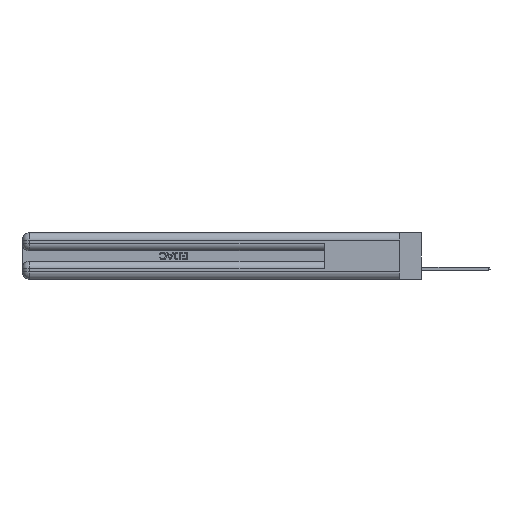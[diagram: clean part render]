
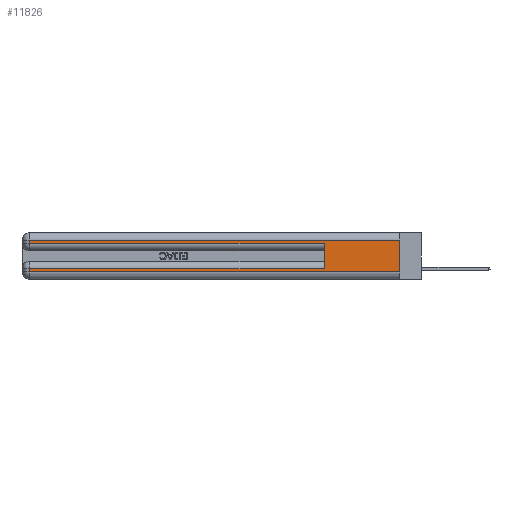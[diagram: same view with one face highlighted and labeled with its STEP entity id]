
A CAD part, left-side view. The second image highlights one B-rep face of the part: STEP entity #11826.
In plain terms, the highlighted planar face has unit normal (-1, 0, 0).
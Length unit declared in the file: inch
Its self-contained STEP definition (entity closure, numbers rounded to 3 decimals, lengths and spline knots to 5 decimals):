
#7 = VECTOR ( 'NONE', #46256, 39.37008 ) ;
#657 = VERTEX_POINT ( 'NONE', #34122 ) ;
#1101 = VECTOR ( 'NONE', #44499, 39.37008 ) ;
#2523 = EDGE_LOOP ( 'NONE', ( #15719, #14985, #14966, #12676, #46068, #41297, #9200, #43063 ) ) ;
#3746 = CARTESIAN_POINT ( 'NONE',  ( 0., 2.94, 0.37 ) ) ;
#4333 = CARTESIAN_POINT ( 'NONE',  ( 0., 0.6, 0.145 ) ) ;
#4435 = VECTOR ( 'NONE', #31436, 39.37008 ) ;
#6180 = VECTOR ( 'NONE', #40109, 39.37008 ) ;
#6723 = VERTEX_POINT ( 'NONE', #40506 ) ;
#6785 = DIRECTION ( 'NONE',  ( 1., 0., 0. ) ) ;
#7247 = CARTESIAN_POINT ( 'NONE',  ( 0., 0., 0.285 ) ) ;
#8791 = CARTESIAN_POINT ( 'NONE',  ( 0., 0.6, 0.285 ) ) ;
#9200 = ORIENTED_EDGE ( 'NONE', *, *, #17586, .T. ) ;
#10290 = CARTESIAN_POINT ( 'NONE',  ( 0., 2.94, 0.37 ) ) ;
#10808 = EDGE_CURVE ( 'NONE', #46349, #21375, #18232, .T. ) ;
#11057 = DIRECTION ( 'NONE',  ( 0., -1., 0. ) ) ;
#11526 = AXIS2_PLACEMENT_3D ( 'NONE', #44281, #6785, #19228 ) ;
#11826 = ADVANCED_FACE ( 'NONE', ( #45069 ), #40083, .F. ) ;
#12674 = CARTESIAN_POINT ( 'NONE',  ( 0., 0., 0.37 ) ) ;
#12676 = ORIENTED_EDGE ( 'NONE', *, *, #21473, .T. ) ;
#13529 = CARTESIAN_POINT ( 'NONE',  ( 0., 0., 0.31 ) ) ;
#14966 = ORIENTED_EDGE ( 'NONE', *, *, #46857, .T. ) ;
#14985 = ORIENTED_EDGE ( 'NONE', *, *, #49122, .T. ) ;
#15719 = ORIENTED_EDGE ( 'NONE', *, *, #10808, .F. ) ;
#16898 = LINE ( 'NONE', #32033, #4435 ) ;
#17586 = EDGE_CURVE ( 'NONE', #51857, #6723, #37594, .T. ) ;
#18232 = LINE ( 'NONE', #12674, #7 ) ;
#18867 = CARTESIAN_POINT ( 'NONE',  ( 0., 2.94, 0.31 ) ) ;
#19228 = DIRECTION ( 'NONE',  ( 0., 0., -1. ) ) ;
#21375 = VERTEX_POINT ( 'NONE', #40155 ) ;
#21473 = EDGE_CURVE ( 'NONE', #45575, #36614, #45914, .T. ) ;
#22296 = EDGE_CURVE ( 'NONE', #6723, #21375, #43138, .T. ) ;
#23285 = LINE ( 'NONE', #23460, #6180 ) ;
#23460 = CARTESIAN_POINT ( 'NONE',  ( 0., 0., 0.31 ) ) ;
#25037 = LINE ( 'NONE', #4333, #49140 ) ;
#25168 = DIRECTION ( 'NONE',  ( 0., 0., -1. ) ) ;
#30613 = VECTOR ( 'NONE', #39414, 39.37008 ) ;
#31436 = DIRECTION ( 'NONE',  ( 0., 1., 0. ) ) ;
#32033 = CARTESIAN_POINT ( 'NONE',  ( 0., 0., 0.085 ) ) ;
#34122 = CARTESIAN_POINT ( 'NONE',  ( 0., 0.6, 0.085 ) ) ;
#35729 = CARTESIAN_POINT ( 'NONE',  ( 0., 0., 0.06 ) ) ;
#36614 = VERTEX_POINT ( 'NONE', #8791 ) ;
#37306 = CARTESIAN_POINT ( 'NONE',  ( 0., 2.94, 0.285 ) ) ;
#37594 = LINE ( 'NONE', #3746, #42109 ) ;
#39414 = DIRECTION ( 'NONE',  ( 0., 0., -1. ) ) ;
#39832 = EDGE_CURVE ( 'NONE', #657, #36614, #25037, .T. ) ;
#40083 = PLANE ( 'NONE',  #11526 ) ;
#40109 = DIRECTION ( 'NONE',  ( 0., 1., 0. ) ) ;
#40155 = CARTESIAN_POINT ( 'NONE',  ( 0., 0., 0.06 ) ) ;
#40506 = CARTESIAN_POINT ( 'NONE',  ( 0., 2.94, 0.06 ) ) ;
#41127 = CARTESIAN_POINT ( 'NONE',  ( 0., 2.94, 0.085 ) ) ;
#41297 = ORIENTED_EDGE ( 'NONE', *, *, #41878, .T. ) ;
#41878 = EDGE_CURVE ( 'NONE', #657, #51857, #16898, .T. ) ;
#42109 = VECTOR ( 'NONE', #25168, 39.37008 ) ;
#43063 = ORIENTED_EDGE ( 'NONE', *, *, #22296, .T. ) ;
#43138 = LINE ( 'NONE', #35729, #1101 ) ;
#44281 = CARTESIAN_POINT ( 'NONE',  ( 0., 0., 0.37 ) ) ;
#44499 = DIRECTION ( 'NONE',  ( 0., -1., 0. ) ) ;
#45069 = FACE_OUTER_BOUND ( 'NONE', #2523, .T. ) ;
#45324 = VECTOR ( 'NONE', #11057, 39.37008 ) ;
#45575 = VERTEX_POINT ( 'NONE', #37306 ) ;
#45914 = LINE ( 'NONE', #7247, #45324 ) ;
#46068 = ORIENTED_EDGE ( 'NONE', *, *, #39832, .F. ) ;
#46256 = DIRECTION ( 'NONE',  ( 0., 0., -1. ) ) ;
#46349 = VERTEX_POINT ( 'NONE', #13529 ) ;
#46857 = EDGE_CURVE ( 'NONE', #50940, #45575, #46903, .T. ) ;
#46903 = LINE ( 'NONE', #10290, #30613 ) ;
#49122 = EDGE_CURVE ( 'NONE', #46349, #50940, #23285, .T. ) ;
#49140 = VECTOR ( 'NONE', #51946, 39.37008 ) ;
#50940 = VERTEX_POINT ( 'NONE', #18867 ) ;
#51857 = VERTEX_POINT ( 'NONE', #41127 ) ;
#51946 = DIRECTION ( 'NONE',  ( 0., 0., 1. ) ) ;
